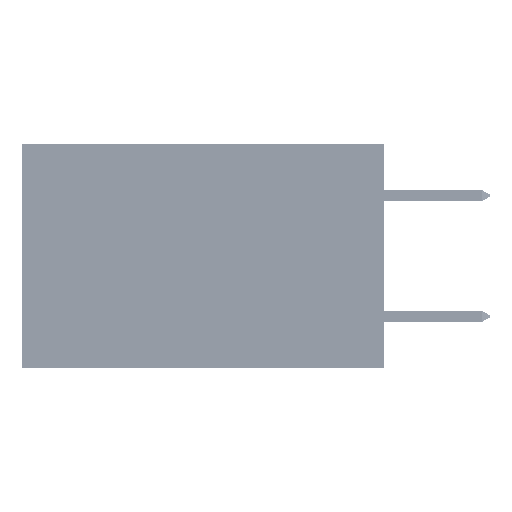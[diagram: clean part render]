
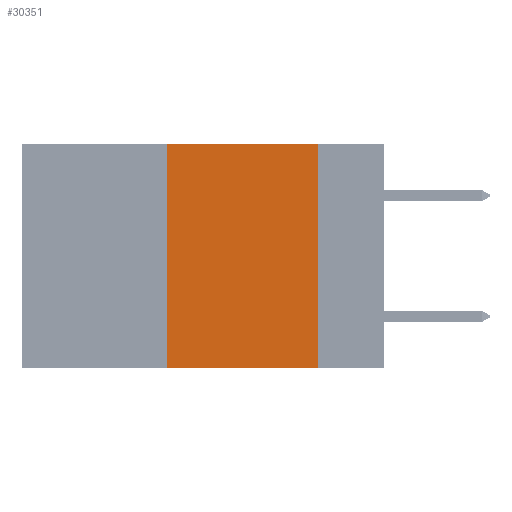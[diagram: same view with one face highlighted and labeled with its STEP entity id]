
A CAD part, left-side view. The second image highlights one B-rep face of the part: STEP entity #30351.
In plain terms, the highlighted planar face has unit normal (-1, 0, 0).
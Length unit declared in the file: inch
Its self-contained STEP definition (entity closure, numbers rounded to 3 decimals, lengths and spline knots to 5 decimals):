
#1627 = CARTESIAN_POINT ( 'NONE',  ( 0., 0.36, 0. ) ) ;
#1989 = ORIENTED_EDGE ( 'NONE', *, *, #23123, .T. ) ;
#4474 = EDGE_CURVE ( 'NONE', #40684, #34804, #24365, .T. ) ;
#5392 = DIRECTION ( 'NONE',  ( 0., 0., 1. ) ) ;
#6279 = DIRECTION ( 'NONE',  ( 0., 0., -1. ) ) ;
#8364 = VERTEX_POINT ( 'NONE', #1627 ) ;
#8918 = CARTESIAN_POINT ( 'NONE',  ( 0., 0.36, 0. ) ) ;
#9361 = CARTESIAN_POINT ( 'NONE',  ( 0., 0.36, -0.37 ) ) ;
#17064 = ORIENTED_EDGE ( 'NONE', *, *, #4474, .F. ) ;
#18243 = CARTESIAN_POINT ( 'NONE',  ( 0., 0.11, -0.37 ) ) ;
#20470 = LINE ( 'NONE', #28018, #37544 ) ;
#23123 = EDGE_CURVE ( 'NONE', #44354, #34804, #41707, .T. ) ;
#24365 = LINE ( 'NONE', #32699, #38723 ) ;
#25436 = DIRECTION ( 'NONE',  ( 1., 0., 0. ) ) ;
#26500 = DIRECTION ( 'NONE',  ( 0., -1., 0. ) ) ;
#26763 = CARTESIAN_POINT ( 'NONE',  ( 0., 0.6, -0.37 ) ) ;
#28018 = CARTESIAN_POINT ( 'NONE',  ( 0., 0.6, 0. ) ) ;
#29610 = ORIENTED_EDGE ( 'NONE', *, *, #33286, .F. ) ;
#30351 = ADVANCED_FACE ( 'NONE', ( #48731 ), #40134, .F. ) ;
#32183 = DIRECTION ( 'NONE',  ( 0., 0., -1. ) ) ;
#32699 = CARTESIAN_POINT ( 'NONE',  ( 0., 0.11, 0. ) ) ;
#33286 = EDGE_CURVE ( 'NONE', #44354, #8364, #35702, .T. ) ;
#34804 = VERTEX_POINT ( 'NONE', #18243 ) ;
#35702 = LINE ( 'NONE', #8918, #39147 ) ;
#36103 = ORIENTED_EDGE ( 'NONE', *, *, #38682, .F. ) ;
#36491 = CARTESIAN_POINT ( 'NONE',  ( 0., 0.11, 0. ) ) ;
#37351 = AXIS2_PLACEMENT_3D ( 'NONE', #44683, #25436, #6279 ) ;
#37544 = VECTOR ( 'NONE', #39690, 39.37008 ) ;
#38682 = EDGE_CURVE ( 'NONE', #8364, #40684, #20470, .T. ) ;
#38723 = VECTOR ( 'NONE', #32183, 39.37008 ) ;
#39147 = VECTOR ( 'NONE', #5392, 39.37008 ) ;
#39175 = EDGE_LOOP ( 'NONE', ( #17064, #36103, #29610, #1989 ) ) ;
#39690 = DIRECTION ( 'NONE',  ( 0., -1., 0. ) ) ;
#40134 = PLANE ( 'NONE',  #37351 ) ;
#40684 = VERTEX_POINT ( 'NONE', #36491 ) ;
#41707 = LINE ( 'NONE', #26763, #49726 ) ;
#44354 = VERTEX_POINT ( 'NONE', #9361 ) ;
#44683 = CARTESIAN_POINT ( 'NONE',  ( 0., 0.6, 0. ) ) ;
#48731 = FACE_OUTER_BOUND ( 'NONE', #39175, .T. ) ;
#49726 = VECTOR ( 'NONE', #26500, 39.37008 ) ;
